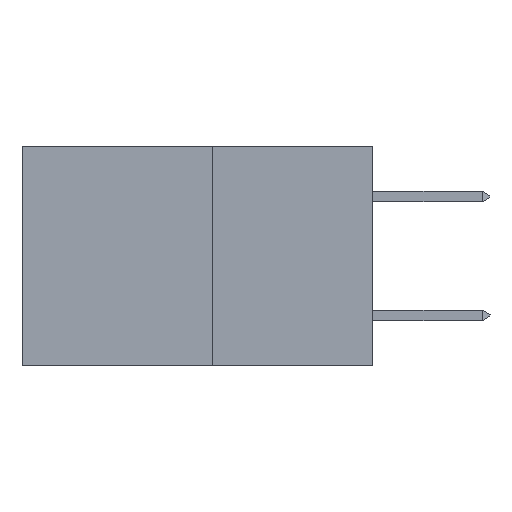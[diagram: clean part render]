
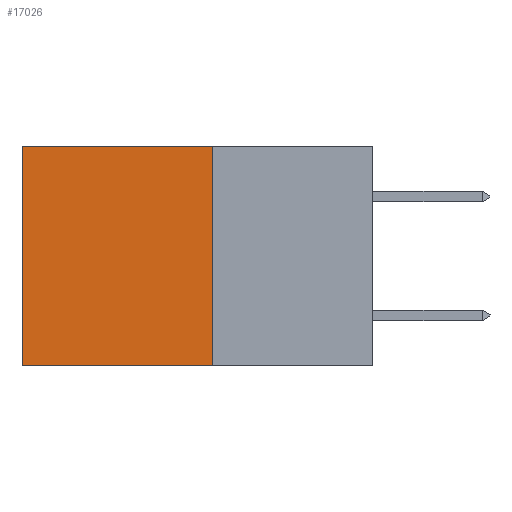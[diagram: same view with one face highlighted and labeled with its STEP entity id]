
A CAD part, left-side view. The second image highlights one B-rep face of the part: STEP entity #17026.
In plain terms, the highlighted planar face has unit normal (-1, 0, 0).
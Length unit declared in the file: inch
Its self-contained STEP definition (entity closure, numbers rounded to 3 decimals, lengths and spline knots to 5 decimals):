
#1113 = CARTESIAN_POINT ( 'NONE',  ( 0.277, 0.27, -0.37 ) ) ;
#2155 = LINE ( 'NONE', #24938, #9249 ) ;
#2399 = ORIENTED_EDGE ( 'NONE', *, *, #29177, .F. ) ;
#2406 = CARTESIAN_POINT ( 'NONE',  ( 0.277, 0.27, -0.37 ) ) ;
#2568 = ORIENTED_EDGE ( 'NONE', *, *, #23489, .T. ) ;
#3138 = VECTOR ( 'NONE', #15390, 39.37008 ) ;
#3333 = EDGE_CURVE ( 'NONE', #15541, #9351, #21350, .T. ) ;
#4109 = AXIS2_PLACEMENT_3D ( 'NONE', #17517, #27073, #12839 ) ;
#4287 = CARTESIAN_POINT ( 'NONE',  ( 0.277, 0.27, 0. ) ) ;
#5673 = VERTEX_POINT ( 'NONE', #23670 ) ;
#6681 = DIRECTION ( 'NONE',  ( 0., 1., 0. ) ) ;
#7036 = VECTOR ( 'NONE', #19027, 39.37008 ) ;
#9249 = VECTOR ( 'NONE', #27333, 39.37008 ) ;
#9351 = VERTEX_POINT ( 'NONE', #10920 ) ;
#10470 = PLANE ( 'NONE',  #4109 ) ;
#10920 = CARTESIAN_POINT ( 'NONE',  ( 0.277, 0.59, -0.37 ) ) ;
#12839 = DIRECTION ( 'NONE',  ( 0., 0., -1. ) ) ;
#13649 = LINE ( 'NONE', #4287, #25543 ) ;
#15390 = DIRECTION ( 'NONE',  ( 0., 0., -1. ) ) ;
#15541 = VERTEX_POINT ( 'NONE', #30698 ) ;
#16491 = CARTESIAN_POINT ( 'NONE',  ( 0.277, 0.59, -0.37 ) ) ;
#17026 = ADVANCED_FACE ( 'NONE', ( #30705 ), #10470, .F. ) ;
#17438 = LINE ( 'NONE', #2406, #7036 ) ;
#17517 = CARTESIAN_POINT ( 'NONE',  ( 0.277, 0.27, -0.37 ) ) ;
#18170 = EDGE_LOOP ( 'NONE', ( #19183, #2399, #21031, #2568 ) ) ;
#19027 = DIRECTION ( 'NONE',  ( 0., 1., 0. ) ) ;
#19183 = ORIENTED_EDGE ( 'NONE', *, *, #3333, .T. ) ;
#21031 = ORIENTED_EDGE ( 'NONE', *, *, #29500, .F. ) ;
#21350 = LINE ( 'NONE', #16491, #3138 ) ;
#23489 = EDGE_CURVE ( 'NONE', #5673, #15541, #13649, .T. ) ;
#23670 = CARTESIAN_POINT ( 'NONE',  ( 0.277, 0.27, 0. ) ) ;
#24583 = VERTEX_POINT ( 'NONE', #1113 ) ;
#24938 = CARTESIAN_POINT ( 'NONE',  ( 0.277, 0.27, -0.37 ) ) ;
#25543 = VECTOR ( 'NONE', #6681, 39.37008 ) ;
#27073 = DIRECTION ( 'NONE',  ( 1., 0., 0. ) ) ;
#27333 = DIRECTION ( 'NONE',  ( 0., 0., -1. ) ) ;
#29177 = EDGE_CURVE ( 'NONE', #24583, #9351, #17438, .T. ) ;
#29500 = EDGE_CURVE ( 'NONE', #5673, #24583, #2155, .T. ) ;
#30698 = CARTESIAN_POINT ( 'NONE',  ( 0.277, 0.59, 0. ) ) ;
#30705 = FACE_OUTER_BOUND ( 'NONE', #18170, .T. ) ;
